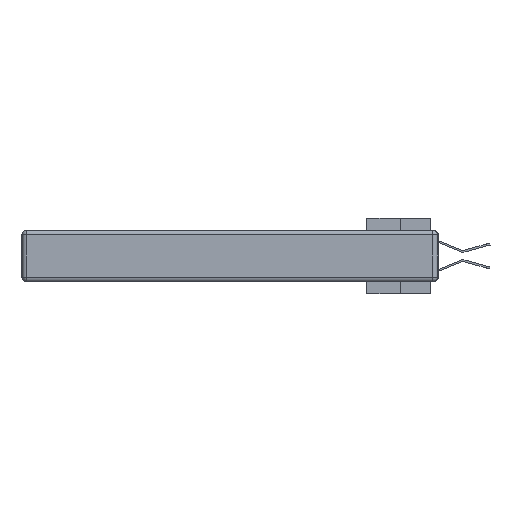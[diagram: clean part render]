
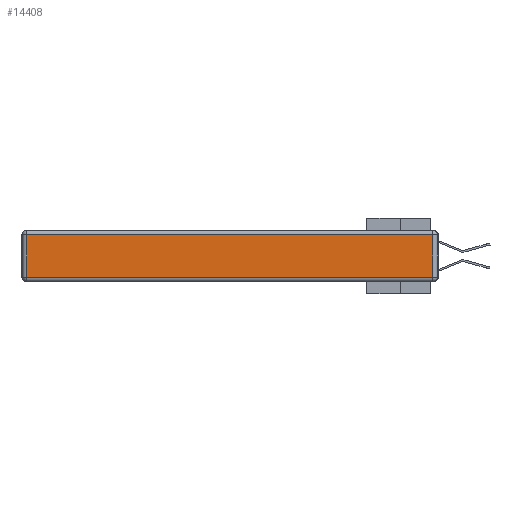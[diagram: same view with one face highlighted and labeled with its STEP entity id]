
A CAD part, left-side view. The second image highlights one B-rep face of the part: STEP entity #14408.
In plain terms, the highlighted planar face has unit normal (-1, 0, 0).
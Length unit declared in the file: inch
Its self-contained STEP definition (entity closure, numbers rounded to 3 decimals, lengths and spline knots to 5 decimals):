
#180 = VECTOR ( 'NONE', #2645, 39.37008 ) ;
#628 = LINE ( 'NONE', #14755, #17731 ) ;
#1407 = EDGE_CURVE ( 'NONE', #12674, #34000, #27190, .T. ) ;
#2290 = LINE ( 'NONE', #13768, #180 ) ;
#2645 = DIRECTION ( 'NONE',  ( 0., 0., -1. ) ) ;
#4251 = FACE_OUTER_BOUND ( 'NONE', #35842, .T. ) ;
#9911 = CARTESIAN_POINT ( 'NONE',  ( 0., 0., -0.343 ) ) ;
#11135 = DIRECTION ( 'NONE',  ( 0., 1., 0. ) ) ;
#11505 = CARTESIAN_POINT ( 'NONE',  ( 0., 2.75, -0.03 ) ) ;
#12674 = VERTEX_POINT ( 'NONE', #20044 ) ;
#12755 = EDGE_CURVE ( 'NONE', #35829, #12674, #628, .T. ) ;
#13768 = CARTESIAN_POINT ( 'NONE',  ( 0., 2.72, -0.343 ) ) ;
#13925 = VERTEX_POINT ( 'NONE', #18796 ) ;
#14408 = ADVANCED_FACE ( 'NONE', ( #4251 ), #30899, .T. ) ;
#14755 = CARTESIAN_POINT ( 'NONE',  ( 0., 0., -0.313 ) ) ;
#16073 = VECTOR ( 'NONE', #23818, 39.37008 ) ;
#17731 = VECTOR ( 'NONE', #26247, 39.37008 ) ;
#17894 = ORIENTED_EDGE ( 'NONE', *, *, #12755, .T. ) ;
#18796 = CARTESIAN_POINT ( 'NONE',  ( 0., 2.72, -0.03 ) ) ;
#18850 = CARTESIAN_POINT ( 'NONE',  ( 0., 0.03, -0.03 ) ) ;
#19955 = ORIENTED_EDGE ( 'NONE', *, *, #1407, .T. ) ;
#20044 = CARTESIAN_POINT ( 'NONE',  ( 0., 0.03, -0.313 ) ) ;
#21390 = DIRECTION ( 'NONE',  ( -1., 0., 0. ) ) ;
#21540 = CARTESIAN_POINT ( 'NONE',  ( 0., 0.03, -0.343 ) ) ;
#23212 = AXIS2_PLACEMENT_3D ( 'NONE', #9911, #21390, #32854 ) ;
#23219 = ORIENTED_EDGE ( 'NONE', *, *, #25450, .T. ) ;
#23818 = DIRECTION ( 'NONE',  ( 0., 0., 1. ) ) ;
#25284 = EDGE_CURVE ( 'NONE', #13925, #35829, #2290, .T. ) ;
#25450 = EDGE_CURVE ( 'NONE', #34000, #13925, #36887, .T. ) ;
#26247 = DIRECTION ( 'NONE',  ( 0., -1., 0. ) ) ;
#27190 = LINE ( 'NONE', #21540, #16073 ) ;
#30104 = VECTOR ( 'NONE', #11135, 39.37008 ) ;
#30899 = PLANE ( 'NONE',  #23212 ) ;
#32854 = DIRECTION ( 'NONE',  ( 0., 0., 1. ) ) ;
#34000 = VERTEX_POINT ( 'NONE', #18850 ) ;
#35271 = CARTESIAN_POINT ( 'NONE',  ( 0., 2.72, -0.313 ) ) ;
#35829 = VERTEX_POINT ( 'NONE', #35271 ) ;
#35842 = EDGE_LOOP ( 'NONE', ( #17894, #19955, #23219, #36650 ) ) ;
#36650 = ORIENTED_EDGE ( 'NONE', *, *, #25284, .T. ) ;
#36887 = LINE ( 'NONE', #11505, #30104 ) ;
